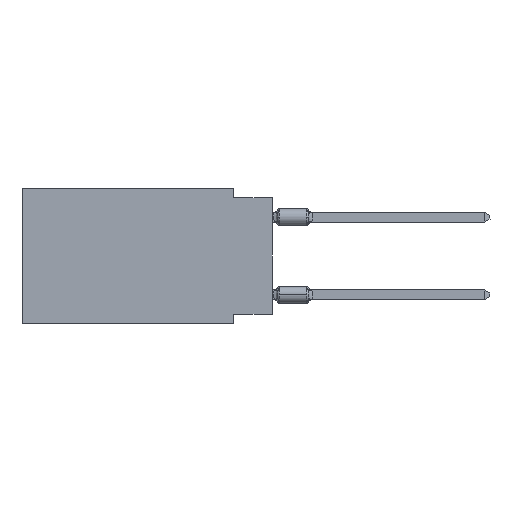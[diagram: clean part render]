
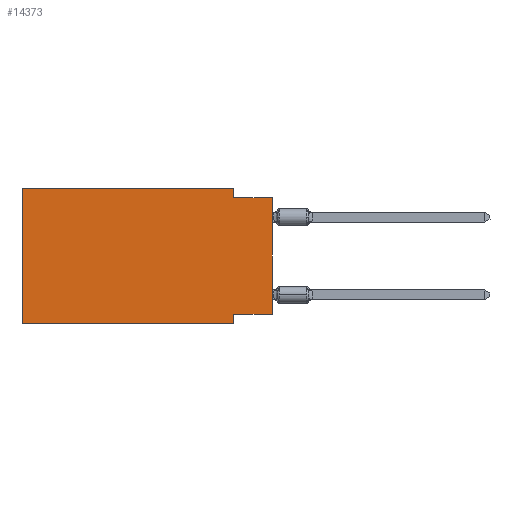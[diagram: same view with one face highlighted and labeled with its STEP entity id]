
A CAD part, left-side view. The second image highlights one B-rep face of the part: STEP entity #14373.
In plain terms, the highlighted planar face has unit normal (-1, 0, 0).
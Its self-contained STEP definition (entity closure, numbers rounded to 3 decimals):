
#71 = CARTESIAN_POINT ( 'NONE',  ( 0., 2.54, -8.89 ) ) ;
#282 = CARTESIAN_POINT ( 'NONE',  ( 0., 2.54, -8.255 ) ) ;
#329 = CARTESIAN_POINT ( 'NONE',  ( 0., 0., -0.635 ) ) ;
#489 = VERTEX_POINT ( 'NONE', #71 ) ;
#669 = CARTESIAN_POINT ( 'NONE',  ( 0., 0., -8.255 ) ) ;
#686 = EDGE_CURVE ( 'NONE', #929, #14408, #5553, .T. ) ;
#929 = VERTEX_POINT ( 'NONE', #3862 ) ;
#958 = LINE ( 'NONE', #9114, #3928 ) ;
#1222 = CARTESIAN_POINT ( 'NONE',  ( 0., 16.383, 0. ) ) ;
#1300 = VERTEX_POINT ( 'NONE', #10552 ) ;
#1348 = CARTESIAN_POINT ( 'NONE',  ( 0., 16.383, 0. ) ) ;
#1369 = LINE ( 'NONE', #7299, #10153 ) ;
#1395 = LINE ( 'NONE', #1608, #9027 ) ;
#1608 = CARTESIAN_POINT ( 'NONE',  ( 0., 0., 0. ) ) ;
#1923 = CARTESIAN_POINT ( 'NONE',  ( 0., 16.383, -8.89 ) ) ;
#3862 = CARTESIAN_POINT ( 'NONE',  ( 0., 0., -8.255 ) ) ;
#3928 = VECTOR ( 'NONE', #12233, 1000. ) ;
#4008 = EDGE_CURVE ( 'NONE', #7220, #7050, #13867, .T. ) ;
#4246 = ORIENTED_EDGE ( 'NONE', *, *, #13631, .F. ) ;
#4349 = ORIENTED_EDGE ( 'NONE', *, *, #4504, .F. ) ;
#4384 = ORIENTED_EDGE ( 'NONE', *, *, #8697, .T. ) ;
#4504 = EDGE_CURVE ( 'NONE', #7050, #1300, #5072, .T. ) ;
#4644 = VERTEX_POINT ( 'NONE', #10320 ) ;
#4853 = CARTESIAN_POINT ( 'NONE',  ( 0., 2.54, 0. ) ) ;
#5039 = ORIENTED_EDGE ( 'NONE', *, *, #9271, .F. ) ;
#5072 = LINE ( 'NONE', #4853, #14159 ) ;
#5163 = ORIENTED_EDGE ( 'NONE', *, *, #11507, .F. ) ;
#5244 = DIRECTION ( 'NONE',  ( 0., 1., 0. ) ) ;
#5382 = VECTOR ( 'NONE', #5244, 1000. ) ;
#5553 = LINE ( 'NONE', #669, #5382 ) ;
#6046 = DIRECTION ( 'NONE',  ( 0., 0., 1. ) ) ;
#6419 = AXIS2_PLACEMENT_3D ( 'NONE', #1348, #10651, #13076 ) ;
#6496 = VECTOR ( 'NONE', #12200, 1000. ) ;
#6502 = ORIENTED_EDGE ( 'NONE', *, *, #4008, .F. ) ;
#7050 = VERTEX_POINT ( 'NONE', #12759 ) ;
#7148 = ORIENTED_EDGE ( 'NONE', *, *, #686, .F. ) ;
#7220 = VERTEX_POINT ( 'NONE', #12366 ) ;
#7299 = CARTESIAN_POINT ( 'NONE',  ( 0., 16.383, -8.89 ) ) ;
#7520 = ORIENTED_EDGE ( 'NONE', *, *, #11775, .T. ) ;
#8339 = LINE ( 'NONE', #13200, #14903 ) ;
#8519 = VERTEX_POINT ( 'NONE', #1923 ) ;
#8697 = EDGE_CURVE ( 'NONE', #929, #4644, #1395, .T. ) ;
#8708 = DIRECTION ( 'NONE',  ( 0., 0., 1. ) ) ;
#9027 = VECTOR ( 'NONE', #6046, 1000. ) ;
#9114 = CARTESIAN_POINT ( 'NONE',  ( 0., 2.54, -8.89 ) ) ;
#9271 = EDGE_CURVE ( 'NONE', #14408, #489, #958, .T. ) ;
#9570 = DIRECTION ( 'NONE',  ( 0., 0., -1. ) ) ;
#10153 = VECTOR ( 'NONE', #10741, 1000. ) ;
#10320 = CARTESIAN_POINT ( 'NONE',  ( 0., 0., -0.635 ) ) ;
#10552 = CARTESIAN_POINT ( 'NONE',  ( 0., 2.54, -0.635 ) ) ;
#10651 = DIRECTION ( 'NONE',  ( 1., 0., 0. ) ) ;
#10741 = DIRECTION ( 'NONE',  ( 0., -1., 0. ) ) ;
#11067 = LINE ( 'NONE', #329, #6496 ) ;
#11507 = EDGE_CURVE ( 'NONE', #1300, #4644, #11067, .T. ) ;
#11598 = DIRECTION ( 'NONE',  ( 0., -1., 0. ) ) ;
#11775 = EDGE_CURVE ( 'NONE', #8519, #489, #1369, .T. ) ;
#12200 = DIRECTION ( 'NONE',  ( 0., -1., 0. ) ) ;
#12233 = DIRECTION ( 'NONE',  ( 0., 0., -1. ) ) ;
#12366 = CARTESIAN_POINT ( 'NONE',  ( 0., 16.383, 0. ) ) ;
#12759 = CARTESIAN_POINT ( 'NONE',  ( 0., 2.54, 0. ) ) ;
#12850 = EDGE_LOOP ( 'NONE', ( #4384, #5163, #4349, #6502, #4246, #7520, #5039, #7148 ) ) ;
#12925 = PLANE ( 'NONE',  #6419 ) ;
#13076 = DIRECTION ( 'NONE',  ( 0., 0., -1. ) ) ;
#13200 = CARTESIAN_POINT ( 'NONE',  ( 0., 16.383, 0. ) ) ;
#13567 = VECTOR ( 'NONE', #11598, 1000. ) ;
#13631 = EDGE_CURVE ( 'NONE', #8519, #7220, #8339, .T. ) ;
#13867 = LINE ( 'NONE', #1222, #13567 ) ;
#14159 = VECTOR ( 'NONE', #9570, 1000. ) ;
#14286 = FACE_OUTER_BOUND ( 'NONE', #12850, .T. ) ;
#14373 = ADVANCED_FACE ( 'NONE', ( #14286 ), #12925, .F. ) ;
#14408 = VERTEX_POINT ( 'NONE', #282 ) ;
#14903 = VECTOR ( 'NONE', #8708, 1000. ) ;
